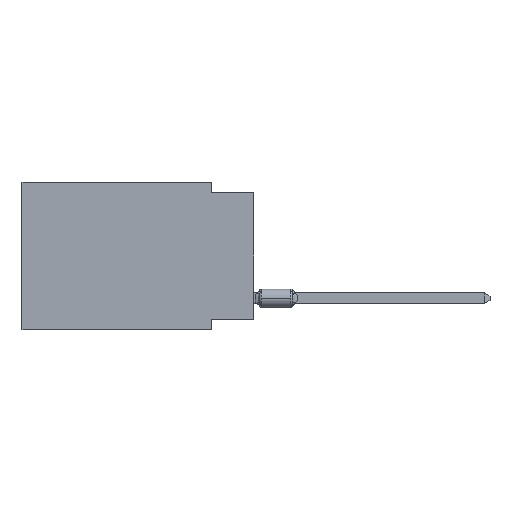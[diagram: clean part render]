
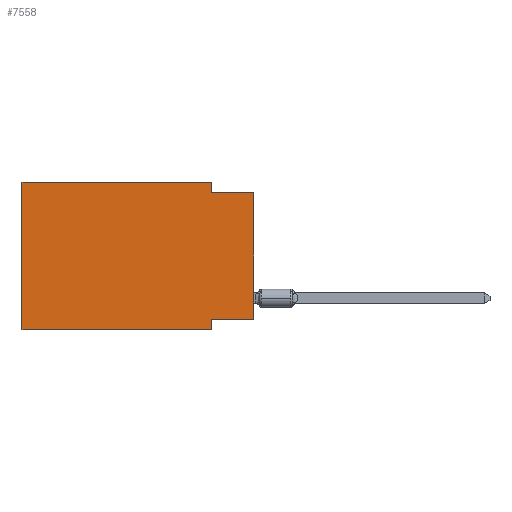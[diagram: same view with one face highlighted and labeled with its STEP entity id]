
A CAD part, left-side view. The second image highlights one B-rep face of the part: STEP entity #7558.
In plain terms, the highlighted planar face has unit normal (-1, 0, 0).
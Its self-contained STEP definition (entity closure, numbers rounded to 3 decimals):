
#607 = FACE_OUTER_BOUND ( 'NONE', #5191, .T. ) ;
#991 = ORIENTED_EDGE ( 'NONE', *, *, #5712, .T. ) ;
#1329 = CARTESIAN_POINT ( 'NONE',  ( 0., 2.54, 0. ) ) ;
#1568 = EDGE_CURVE ( 'NONE', #6585, #20272, #7185, .T. ) ;
#1586 = CARTESIAN_POINT ( 'NONE',  ( 0., 2.54, -8.89 ) ) ;
#1759 = DIRECTION ( 'NONE',  ( 0., 0., -1. ) ) ;
#2259 = VERTEX_POINT ( 'NONE', #11584 ) ;
#2417 = DIRECTION ( 'NONE',  ( 0., 0., -1. ) ) ;
#2447 = CARTESIAN_POINT ( 'NONE',  ( 0., 2.54, -0.635 ) ) ;
#2572 = CARTESIAN_POINT ( 'NONE',  ( 0., 13.97, -8.89 ) ) ;
#2694 = CARTESIAN_POINT ( 'NONE',  ( 0., 0., -8.255 ) ) ;
#2773 = LINE ( 'NONE', #2572, #17430 ) ;
#2953 = LINE ( 'NONE', #9371, #13420 ) ;
#2982 = ORIENTED_EDGE ( 'NONE', *, *, #19221, .F. ) ;
#3539 = LINE ( 'NONE', #8176, #9046 ) ;
#3625 = CARTESIAN_POINT ( 'NONE',  ( 0., 0., -0.635 ) ) ;
#3629 = VECTOR ( 'NONE', #12176, 1000. ) ;
#3844 = DIRECTION ( 'NONE',  ( 0., 1., 0. ) ) ;
#4070 = CARTESIAN_POINT ( 'NONE',  ( 0., 13.97, 0. ) ) ;
#5191 = EDGE_LOOP ( 'NONE', ( #10258, #7252, #17572, #2982, #17631, #991, #14368, #18791 ) ) ;
#5433 = AXIS2_PLACEMENT_3D ( 'NONE', #14849, #6928, #2417 ) ;
#5445 = PLANE ( 'NONE',  #5433 ) ;
#5712 = EDGE_CURVE ( 'NONE', #18215, #8633, #2773, .T. ) ;
#5824 = CARTESIAN_POINT ( 'NONE',  ( 0., 13.97, 0. ) ) ;
#6585 = VERTEX_POINT ( 'NONE', #2694 ) ;
#6928 = DIRECTION ( 'NONE',  ( 1., 0., 0. ) ) ;
#6988 = LINE ( 'NONE', #5824, #3629 ) ;
#7109 = VECTOR ( 'NONE', #10250, 1000. ) ;
#7185 = LINE ( 'NONE', #16780, #10032 ) ;
#7252 = ORIENTED_EDGE ( 'NONE', *, *, #14642, .F. ) ;
#7487 = DIRECTION ( 'NONE',  ( 0., 0., 1. ) ) ;
#7558 = ADVANCED_FACE ( 'NONE', ( #607 ), #5445, .F. ) ;
#8176 = CARTESIAN_POINT ( 'NONE',  ( 0., 0., -8.255 ) ) ;
#8402 = CARTESIAN_POINT ( 'NONE',  ( 0., 2.54, -8.255 ) ) ;
#8415 = CARTESIAN_POINT ( 'NONE',  ( 0., 13.97, -8.89 ) ) ;
#8633 = VERTEX_POINT ( 'NONE', #1586 ) ;
#9046 = VECTOR ( 'NONE', #3844, 1000. ) ;
#9371 = CARTESIAN_POINT ( 'NONE',  ( 0., 13.97, 0. ) ) ;
#10032 = VECTOR ( 'NONE', #7487, 1000. ) ;
#10250 = DIRECTION ( 'NONE',  ( 0., 0., -1. ) ) ;
#10258 = ORIENTED_EDGE ( 'NONE', *, *, #1568, .T. ) ;
#10281 = LINE ( 'NONE', #3625, #17484 ) ;
#11584 = CARTESIAN_POINT ( 'NONE',  ( 0., 2.54, 0. ) ) ;
#11840 = CARTESIAN_POINT ( 'NONE',  ( 0., 2.54, -8.89 ) ) ;
#12149 = LINE ( 'NONE', #11840, #7109 ) ;
#12176 = DIRECTION ( 'NONE',  ( 0., -1., 0. ) ) ;
#12437 = VECTOR ( 'NONE', #1759, 1000. ) ;
#12643 = DIRECTION ( 'NONE',  ( 0., 0., 1. ) ) ;
#12776 = VERTEX_POINT ( 'NONE', #2447 ) ;
#12850 = EDGE_CURVE ( 'NONE', #18215, #14477, #2953, .T. ) ;
#13420 = VECTOR ( 'NONE', #12643, 1000. ) ;
#14368 = ORIENTED_EDGE ( 'NONE', *, *, #15243, .F. ) ;
#14477 = VERTEX_POINT ( 'NONE', #4070 ) ;
#14597 = EDGE_CURVE ( 'NONE', #2259, #12776, #16203, .T. ) ;
#14642 = EDGE_CURVE ( 'NONE', #12776, #20272, #10281, .T. ) ;
#14707 = CARTESIAN_POINT ( 'NONE',  ( 0., 0., -0.635 ) ) ;
#14849 = CARTESIAN_POINT ( 'NONE',  ( 0., 13.97, 0. ) ) ;
#15243 = EDGE_CURVE ( 'NONE', #17030, #8633, #12149, .T. ) ;
#16203 = LINE ( 'NONE', #1329, #12437 ) ;
#16392 = DIRECTION ( 'NONE',  ( 0., -1., 0. ) ) ;
#16780 = CARTESIAN_POINT ( 'NONE',  ( 0., 0., 0. ) ) ;
#17030 = VERTEX_POINT ( 'NONE', #8402 ) ;
#17223 = DIRECTION ( 'NONE',  ( 0., -1., 0. ) ) ;
#17430 = VECTOR ( 'NONE', #17223, 1000. ) ;
#17484 = VECTOR ( 'NONE', #16392, 1000. ) ;
#17572 = ORIENTED_EDGE ( 'NONE', *, *, #14597, .F. ) ;
#17631 = ORIENTED_EDGE ( 'NONE', *, *, #12850, .F. ) ;
#18215 = VERTEX_POINT ( 'NONE', #8415 ) ;
#18791 = ORIENTED_EDGE ( 'NONE', *, *, #20306, .F. ) ;
#19221 = EDGE_CURVE ( 'NONE', #14477, #2259, #6988, .T. ) ;
#20272 = VERTEX_POINT ( 'NONE', #14707 ) ;
#20306 = EDGE_CURVE ( 'NONE', #6585, #17030, #3539, .T. ) ;
